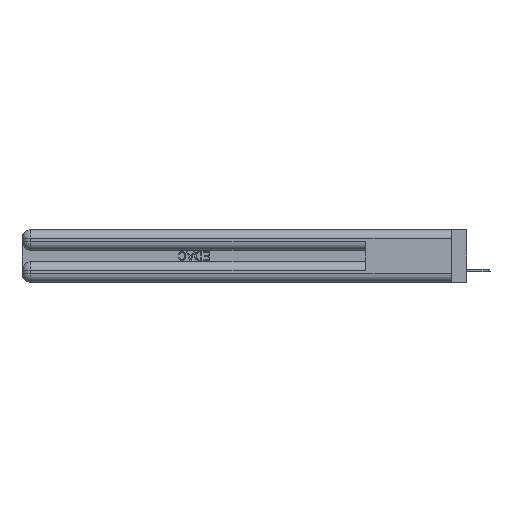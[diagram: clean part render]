
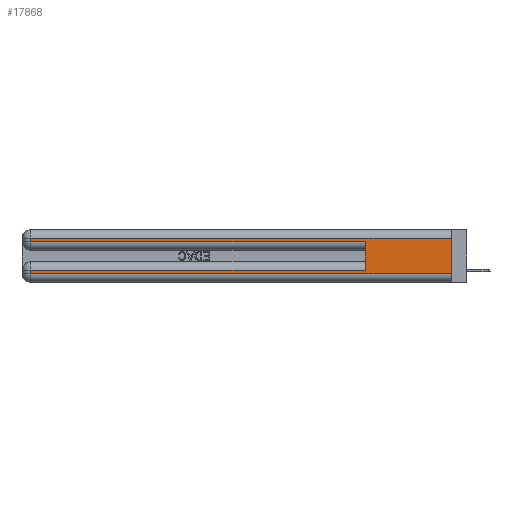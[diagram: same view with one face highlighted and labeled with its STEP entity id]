
A CAD part, left-side view. The second image highlights one B-rep face of the part: STEP entity #17868.
In plain terms, the highlighted planar face has unit normal (-1, 0, 0).
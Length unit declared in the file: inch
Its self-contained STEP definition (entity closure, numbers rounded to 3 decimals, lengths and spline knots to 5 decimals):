
#261 = VECTOR ( 'NONE', #10006, 39.37008 ) ;
#371 = FACE_OUTER_BOUND ( 'NONE', #31394, .T. ) ;
#794 = CARTESIAN_POINT ( 'NONE',  ( 0., 0., 0.31 ) ) ;
#864 = EDGE_CURVE ( 'NONE', #24975, #10388, #7452, .T. ) ;
#1170 = LINE ( 'NONE', #36274, #261 ) ;
#1355 = PLANE ( 'NONE',  #26801 ) ;
#2669 = DIRECTION ( 'NONE',  ( 0., 1., 0. ) ) ;
#2900 = VECTOR ( 'NONE', #26126, 39.37008 ) ;
#3757 = DIRECTION ( 'NONE',  ( 0., 1., 0. ) ) ;
#5462 = CARTESIAN_POINT ( 'NONE',  ( 0., 0., 0.085 ) ) ;
#6286 = LINE ( 'NONE', #5462, #27838 ) ;
#6355 = VERTEX_POINT ( 'NONE', #18473 ) ;
#7452 = LINE ( 'NONE', #32139, #2900 ) ;
#7872 = VERTEX_POINT ( 'NONE', #23002 ) ;
#7991 = ORIENTED_EDGE ( 'NONE', *, *, #17684, .T. ) ;
#8595 = CARTESIAN_POINT ( 'NONE',  ( 0., 0.6, 0.285 ) ) ;
#8815 = LINE ( 'NONE', #794, #18012 ) ;
#9855 = EDGE_CURVE ( 'NONE', #14215, #17246, #29597, .T. ) ;
#10006 = DIRECTION ( 'NONE',  ( 0., 0., 1. ) ) ;
#10197 = EDGE_CURVE ( 'NONE', #7872, #24975, #15024, .T. ) ;
#10388 = VERTEX_POINT ( 'NONE', #8595 ) ;
#10931 = DIRECTION ( 'NONE',  ( 0., 0., -1. ) ) ;
#11697 = VERTEX_POINT ( 'NONE', #37566 ) ;
#11700 = EDGE_CURVE ( 'NONE', #37520, #10388, #1170, .T. ) ;
#12444 = ORIENTED_EDGE ( 'NONE', *, *, #864, .T. ) ;
#13560 = CARTESIAN_POINT ( 'NONE',  ( 0., 0., 0.37 ) ) ;
#13788 = CARTESIAN_POINT ( 'NONE',  ( 0., 2.94, 0.06 ) ) ;
#14215 = VERTEX_POINT ( 'NONE', #13788 ) ;
#15024 = LINE ( 'NONE', #30119, #28709 ) ;
#15967 = DIRECTION ( 'NONE',  ( 1., 0., 0. ) ) ;
#16322 = DIRECTION ( 'NONE',  ( 0., 0., -1. ) ) ;
#17246 = VERTEX_POINT ( 'NONE', #21123 ) ;
#17307 = ORIENTED_EDGE ( 'NONE', *, *, #20712, .T. ) ;
#17684 = EDGE_CURVE ( 'NONE', #37520, #11697, #6286, .T. ) ;
#17868 = ADVANCED_FACE ( 'NONE', ( #371 ), #1355, .F. ) ;
#18012 = VECTOR ( 'NONE', #3757, 39.37008 ) ;
#18473 = CARTESIAN_POINT ( 'NONE',  ( 0., 0., 0.31 ) ) ;
#19557 = CARTESIAN_POINT ( 'NONE',  ( 0., 2.94, 0.37 ) ) ;
#20051 = ORIENTED_EDGE ( 'NONE', *, *, #31197, .F. ) ;
#20454 = VECTOR ( 'NONE', #10931, 39.37008 ) ;
#20712 = EDGE_CURVE ( 'NONE', #6355, #7872, #8815, .T. ) ;
#21123 = CARTESIAN_POINT ( 'NONE',  ( 0., 0., 0.06 ) ) ;
#21903 = VECTOR ( 'NONE', #34193, 39.37008 ) ;
#21939 = DIRECTION ( 'NONE',  ( 0., 0., -1. ) ) ;
#23002 = CARTESIAN_POINT ( 'NONE',  ( 0., 2.94, 0.31 ) ) ;
#24767 = ORIENTED_EDGE ( 'NONE', *, *, #9855, .T. ) ;
#24975 = VERTEX_POINT ( 'NONE', #36408 ) ;
#25572 = ORIENTED_EDGE ( 'NONE', *, *, #34820, .T. ) ;
#25676 = VECTOR ( 'NONE', #25715, 39.37008 ) ;
#25715 = DIRECTION ( 'NONE',  ( 0., 0., -1. ) ) ;
#26126 = DIRECTION ( 'NONE',  ( 0., -1., 0. ) ) ;
#26354 = CARTESIAN_POINT ( 'NONE',  ( 0., 0., 0.37 ) ) ;
#26768 = ORIENTED_EDGE ( 'NONE', *, *, #10197, .T. ) ;
#26801 = AXIS2_PLACEMENT_3D ( 'NONE', #13560, #15967, #21939 ) ;
#27838 = VECTOR ( 'NONE', #2669, 39.37008 ) ;
#28709 = VECTOR ( 'NONE', #16322, 39.37008 ) ;
#29597 = LINE ( 'NONE', #37178, #21903 ) ;
#30119 = CARTESIAN_POINT ( 'NONE',  ( 0., 2.94, 0.37 ) ) ;
#31197 = EDGE_CURVE ( 'NONE', #6355, #17246, #32388, .T. ) ;
#31394 = EDGE_LOOP ( 'NONE', ( #20051, #17307, #26768, #12444, #31918, #7991, #25572, #24767 ) ) ;
#31918 = ORIENTED_EDGE ( 'NONE', *, *, #11700, .F. ) ;
#32139 = CARTESIAN_POINT ( 'NONE',  ( 0., 0., 0.285 ) ) ;
#32388 = LINE ( 'NONE', #26354, #25676 ) ;
#33144 = CARTESIAN_POINT ( 'NONE',  ( 0., 0.6, 0.085 ) ) ;
#34193 = DIRECTION ( 'NONE',  ( 0., -1., 0. ) ) ;
#34820 = EDGE_CURVE ( 'NONE', #11697, #14215, #35748, .T. ) ;
#35748 = LINE ( 'NONE', #19557, #20454 ) ;
#36274 = CARTESIAN_POINT ( 'NONE',  ( 0., 0.6, 0.145 ) ) ;
#36408 = CARTESIAN_POINT ( 'NONE',  ( 0., 2.94, 0.285 ) ) ;
#37178 = CARTESIAN_POINT ( 'NONE',  ( 0., 0., 0.06 ) ) ;
#37520 = VERTEX_POINT ( 'NONE', #33144 ) ;
#37566 = CARTESIAN_POINT ( 'NONE',  ( 0., 2.94, 0.085 ) ) ;
